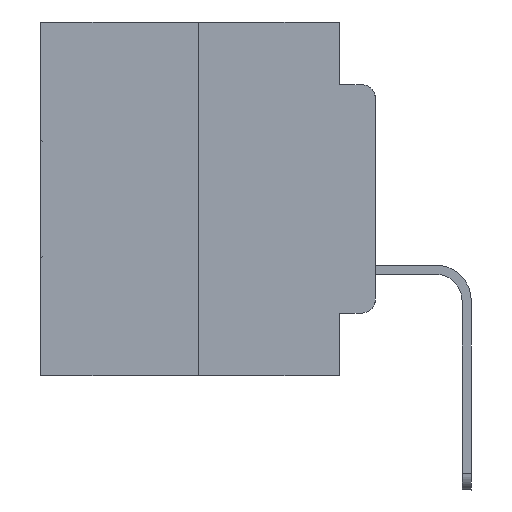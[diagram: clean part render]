
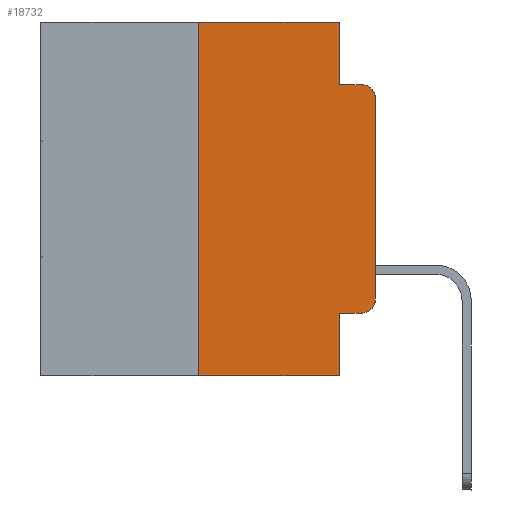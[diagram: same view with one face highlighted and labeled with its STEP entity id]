
A CAD part, left-side view. The second image highlights one B-rep face of the part: STEP entity #18732.
In plain terms, the highlighted planar face has unit normal (-1, 0, 0).
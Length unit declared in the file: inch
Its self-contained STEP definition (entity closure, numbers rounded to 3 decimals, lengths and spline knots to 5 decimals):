
#143 = ORIENTED_EDGE ( 'NONE', *, *, #23730, .T. ) ;
#310 = CIRCLE ( 'NONE', #21940, 0.02 ) ;
#992 = CARTESIAN_POINT ( 'NONE',  ( 0., 0.051, -0.0885 ) ) ;
#1124 = CARTESIAN_POINT ( 'NONE',  ( 0., 0.051, -0.0885 ) ) ;
#1408 = VECTOR ( 'NONE', #11339, 39.37008 ) ;
#1928 = CARTESIAN_POINT ( 'NONE',  ( 0., 0.051, -0.5 ) ) ;
#2148 = VECTOR ( 'NONE', #14708, 39.37008 ) ;
#2272 = VECTOR ( 'NONE', #22658, 39.37008 ) ;
#2529 = CARTESIAN_POINT ( 'NONE',  ( 0., 0.02, -0.4115 ) ) ;
#2649 = ORIENTED_EDGE ( 'NONE', *, *, #26712, .F. ) ;
#3087 = VERTEX_POINT ( 'NONE', #8359 ) ;
#3177 = CARTESIAN_POINT ( 'NONE',  ( 0., 0.02, -0.0885 ) ) ;
#3361 = DIRECTION ( 'NONE',  ( 0., 0., -1. ) ) ;
#3401 = ORIENTED_EDGE ( 'NONE', *, *, #27102, .F. ) ;
#3662 = DIRECTION ( 'NONE',  ( 0., -1., 0. ) ) ;
#3692 = EDGE_CURVE ( 'NONE', #11437, #6046, #310, .T. ) ;
#4239 = CARTESIAN_POINT ( 'NONE',  ( 0., 0.25, 0. ) ) ;
#4280 = VECTOR ( 'NONE', #7101, 39.37008 ) ;
#4460 = CIRCLE ( 'NONE', #7981, 0.02 ) ;
#4648 = PLANE ( 'NONE',  #20182 ) ;
#4749 = DIRECTION ( 'NONE',  ( 1., 0., 0. ) ) ;
#4780 = VERTEX_POINT ( 'NONE', #23333 ) ;
#5040 = DIRECTION ( 'NONE',  ( 0., 0., -1. ) ) ;
#5572 = CARTESIAN_POINT ( 'NONE',  ( 0., 0.02, -0.1085 ) ) ;
#5981 = DIRECTION ( 'NONE',  ( 0., 0., -1. ) ) ;
#6046 = VERTEX_POINT ( 'NONE', #3177 ) ;
#6423 = LINE ( 'NONE', #22474, #11098 ) ;
#7101 = DIRECTION ( 'NONE',  ( 0., 0., -1. ) ) ;
#7330 = LINE ( 'NONE', #4239, #2272 ) ;
#7746 = VERTEX_POINT ( 'NONE', #13185 ) ;
#7981 = AXIS2_PLACEMENT_3D ( 'NONE', #19946, #22199, #5981 ) ;
#8240 = LINE ( 'NONE', #20976, #4280 ) ;
#8242 = LINE ( 'NONE', #16219, #1408 ) ;
#8359 = CARTESIAN_POINT ( 'NONE',  ( 0., 0.25, -0.5 ) ) ;
#9959 = ORIENTED_EDGE ( 'NONE', *, *, #19889, .F. ) ;
#10452 = LINE ( 'NONE', #992, #2148 ) ;
#11098 = VECTOR ( 'NONE', #3662, 39.37008 ) ;
#11339 = DIRECTION ( 'NONE',  ( 0., -1., 0. ) ) ;
#11437 = VERTEX_POINT ( 'NONE', #12913 ) ;
#12581 = CARTESIAN_POINT ( 'NONE',  ( 0., 0., 0. ) ) ;
#12913 = CARTESIAN_POINT ( 'NONE',  ( 0., 0., -0.1085 ) ) ;
#12998 = LINE ( 'NONE', #14227, #14062 ) ;
#13185 = CARTESIAN_POINT ( 'NONE',  ( 0., 0.051, -0.4115 ) ) ;
#13630 = CARTESIAN_POINT ( 'NONE',  ( 0., 0.473, 0. ) ) ;
#13687 = ORIENTED_EDGE ( 'NONE', *, *, #16888, .F. ) ;
#14062 = VECTOR ( 'NONE', #5040, 39.37008 ) ;
#14227 = CARTESIAN_POINT ( 'NONE',  ( 0., 0.051, 0. ) ) ;
#14657 = DIRECTION ( 'NONE',  ( -1., 0., 0. ) ) ;
#14708 = DIRECTION ( 'NONE',  ( 0., -1., 0. ) ) ;
#15129 = VERTEX_POINT ( 'NONE', #1928 ) ;
#16219 = CARTESIAN_POINT ( 'NONE',  ( 0., 0.473, 0. ) ) ;
#16438 = VERTEX_POINT ( 'NONE', #16603 ) ;
#16603 = CARTESIAN_POINT ( 'NONE',  ( 0., 0.051, 0. ) ) ;
#16888 = EDGE_CURVE ( 'NONE', #3087, #29427, #7330, .T. ) ;
#18732 = ADVANCED_FACE ( 'NONE', ( #27481 ), #4648, .F. ) ;
#18756 = VECTOR ( 'NONE', #28635, 39.37008 ) ;
#19260 = VERTEX_POINT ( 'NONE', #2529 ) ;
#19361 = EDGE_CURVE ( 'NONE', #7746, #15129, #12998, .T. ) ;
#19889 = EDGE_CURVE ( 'NONE', #29427, #16438, #8242, .T. ) ;
#19946 = CARTESIAN_POINT ( 'NONE',  ( 0., 0.02, -0.3915 ) ) ;
#20001 = VECTOR ( 'NONE', #27296, 39.37008 ) ;
#20084 = EDGE_CURVE ( 'NONE', #4780, #11437, #22398, .T. ) ;
#20182 = AXIS2_PLACEMENT_3D ( 'NONE', #13630, #4749, #20947 ) ;
#20347 = CARTESIAN_POINT ( 'NONE',  ( 0., 0.473, -0.5 ) ) ;
#20947 = DIRECTION ( 'NONE',  ( 0., 0., -1. ) ) ;
#20976 = CARTESIAN_POINT ( 'NONE',  ( 0., 0.051, 0. ) ) ;
#21260 = EDGE_LOOP ( 'NONE', ( #22263, #25449, #2649, #3401, #9959, #13687, #143, #25122, #25942, #23651 ) ) ;
#21940 = AXIS2_PLACEMENT_3D ( 'NONE', #5572, #14657, #3361 ) ;
#22199 = DIRECTION ( 'NONE',  ( -1., 0., 0. ) ) ;
#22263 = ORIENTED_EDGE ( 'NONE', *, *, #20084, .T. ) ;
#22398 = LINE ( 'NONE', #12581, #18756 ) ;
#22474 = CARTESIAN_POINT ( 'NONE',  ( 0., 0.051, -0.4115 ) ) ;
#22658 = DIRECTION ( 'NONE',  ( 0., 0., 1. ) ) ;
#22912 = CARTESIAN_POINT ( 'NONE',  ( 0., 0.25, 0. ) ) ;
#23333 = CARTESIAN_POINT ( 'NONE',  ( 0., 0., -0.3915 ) ) ;
#23651 = ORIENTED_EDGE ( 'NONE', *, *, #29836, .T. ) ;
#23730 = EDGE_CURVE ( 'NONE', #3087, #15129, #29375, .T. ) ;
#25122 = ORIENTED_EDGE ( 'NONE', *, *, #19361, .F. ) ;
#25449 = ORIENTED_EDGE ( 'NONE', *, *, #3692, .T. ) ;
#25942 = ORIENTED_EDGE ( 'NONE', *, *, #27566, .T. ) ;
#26218 = VERTEX_POINT ( 'NONE', #1124 ) ;
#26712 = EDGE_CURVE ( 'NONE', #26218, #6046, #10452, .T. ) ;
#27102 = EDGE_CURVE ( 'NONE', #16438, #26218, #8240, .T. ) ;
#27296 = DIRECTION ( 'NONE',  ( 0., -1., 0. ) ) ;
#27481 = FACE_OUTER_BOUND ( 'NONE', #21260, .T. ) ;
#27566 = EDGE_CURVE ( 'NONE', #7746, #19260, #6423, .T. ) ;
#28635 = DIRECTION ( 'NONE',  ( 0., 0., 1. ) ) ;
#29375 = LINE ( 'NONE', #20347, #20001 ) ;
#29427 = VERTEX_POINT ( 'NONE', #22912 ) ;
#29836 = EDGE_CURVE ( 'NONE', #19260, #4780, #4460, .T. ) ;
